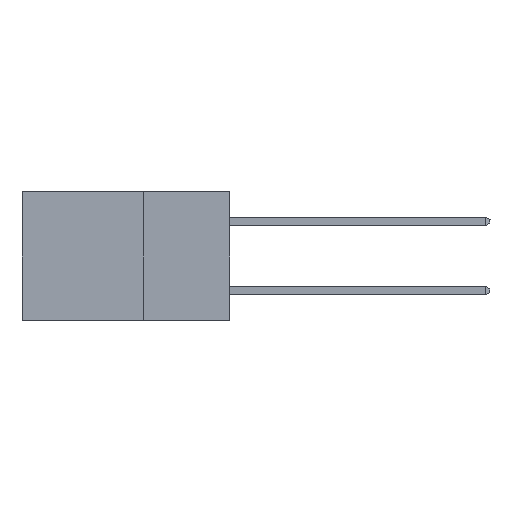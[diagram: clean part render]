
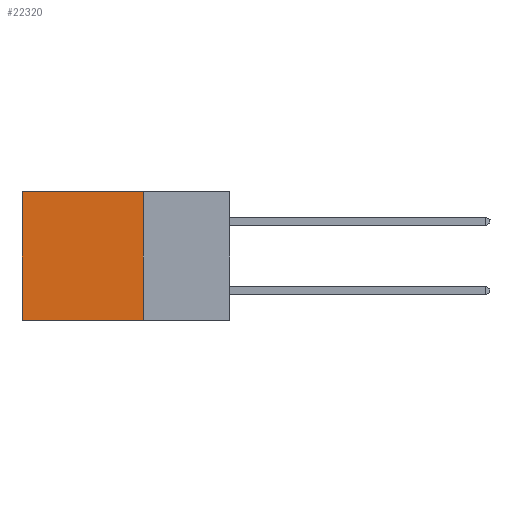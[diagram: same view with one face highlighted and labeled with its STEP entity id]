
A CAD part, left-side view. The second image highlights one B-rep face of the part: STEP entity #22320.
In plain terms, the highlighted planar face has unit normal (-1, 0, 0).
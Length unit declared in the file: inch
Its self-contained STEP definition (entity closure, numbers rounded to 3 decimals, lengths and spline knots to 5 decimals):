
#671 = EDGE_CURVE ( 'NONE', #11178, #15696, #19512, .T. ) ;
#2265 = VERTEX_POINT ( 'NONE', #13654 ) ;
#2779 = VECTOR ( 'NONE', #20730, 39.37008 ) ;
#3317 = VECTOR ( 'NONE', #13407, 39.37008 ) ;
#3936 = DIRECTION ( 'NONE',  ( 0., 1., 0. ) ) ;
#4013 = CARTESIAN_POINT ( 'NONE',  ( 0.2615, 0.25, -0.37 ) ) ;
#4105 = ORIENTED_EDGE ( 'NONE', *, *, #15297, .F. ) ;
#6276 = LINE ( 'NONE', #18817, #2779 ) ;
#6731 = CARTESIAN_POINT ( 'NONE',  ( 0.2615, 0.25, 0. ) ) ;
#6734 = VERTEX_POINT ( 'NONE', #4013 ) ;
#7211 = LINE ( 'NONE', #21661, #3317 ) ;
#7276 = AXIS2_PLACEMENT_3D ( 'NONE', #22133, #22274, #13762 ) ;
#8361 = LINE ( 'NONE', #10282, #9727 ) ;
#9727 = VECTOR ( 'NONE', #3936, 39.37008 ) ;
#10282 = CARTESIAN_POINT ( 'NONE',  ( 0.2615, 0.25, -0.37 ) ) ;
#11178 = VERTEX_POINT ( 'NONE', #17791 ) ;
#13407 = DIRECTION ( 'NONE',  ( 0., 0., -1. ) ) ;
#13654 = CARTESIAN_POINT ( 'NONE',  ( 0.2615, 0.6, -0.37 ) ) ;
#13762 = DIRECTION ( 'NONE',  ( 0., 0., -1. ) ) ;
#14505 = CARTESIAN_POINT ( 'NONE',  ( 0.2615, 0.6, 0. ) ) ;
#15297 = EDGE_CURVE ( 'NONE', #6734, #2265, #8361, .T. ) ;
#15444 = ORIENTED_EDGE ( 'NONE', *, *, #21118, .F. ) ;
#15696 = VERTEX_POINT ( 'NONE', #14505 ) ;
#16268 = EDGE_LOOP ( 'NONE', ( #19619, #4105, #15444, #26627 ) ) ;
#17791 = CARTESIAN_POINT ( 'NONE',  ( 0.2615, 0.25, 0. ) ) ;
#18680 = VECTOR ( 'NONE', #19656, 39.37008 ) ;
#18817 = CARTESIAN_POINT ( 'NONE',  ( 0.2615, 0.25, -0.37 ) ) ;
#19512 = LINE ( 'NONE', #6731, #18680 ) ;
#19619 = ORIENTED_EDGE ( 'NONE', *, *, #22584, .T. ) ;
#19656 = DIRECTION ( 'NONE',  ( 0., 1., 0. ) ) ;
#20730 = DIRECTION ( 'NONE',  ( 0., 0., -1. ) ) ;
#21118 = EDGE_CURVE ( 'NONE', #11178, #6734, #6276, .T. ) ;
#21661 = CARTESIAN_POINT ( 'NONE',  ( 0.2615, 0.6, -0.37 ) ) ;
#21863 = PLANE ( 'NONE',  #7276 ) ;
#22133 = CARTESIAN_POINT ( 'NONE',  ( 0.2615, 0.25, -0.37 ) ) ;
#22274 = DIRECTION ( 'NONE',  ( 1., 0., 0. ) ) ;
#22320 = ADVANCED_FACE ( 'NONE', ( #26434 ), #21863, .F. ) ;
#22584 = EDGE_CURVE ( 'NONE', #15696, #2265, #7211, .T. ) ;
#26434 = FACE_OUTER_BOUND ( 'NONE', #16268, .T. ) ;
#26627 = ORIENTED_EDGE ( 'NONE', *, *, #671, .T. ) ;
